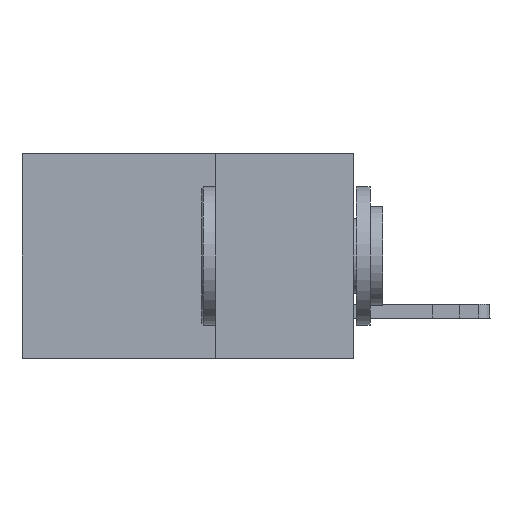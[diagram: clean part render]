
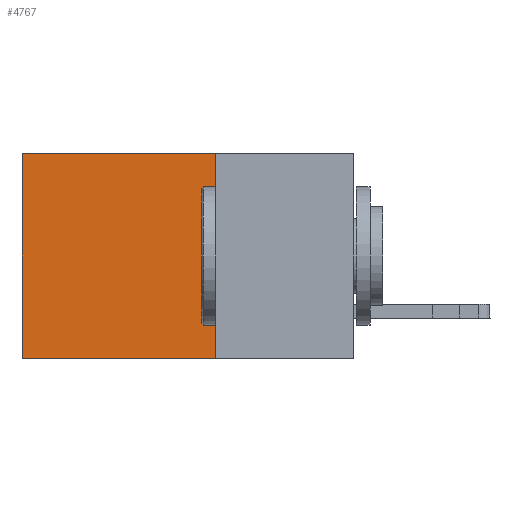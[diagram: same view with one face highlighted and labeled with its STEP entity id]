
A CAD part, left-side view. The second image highlights one B-rep face of the part: STEP entity #4767.
In plain terms, the highlighted planar face has unit normal (-1, 0, 0).
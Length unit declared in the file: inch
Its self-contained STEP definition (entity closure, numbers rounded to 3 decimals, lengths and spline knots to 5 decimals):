
#825 = VERTEX_POINT ( 'NONE', #21535 ) ;
#1037 = DIRECTION ( 'NONE',  ( 1., 0., 0. ) ) ;
#1356 = DIRECTION ( 'NONE',  ( 0., 0., -1. ) ) ;
#3114 = VECTOR ( 'NONE', #20993, 39.37008 ) ;
#3128 = PLANE ( 'NONE',  #12236 ) ;
#3600 = CARTESIAN_POINT ( 'NONE',  ( 0.2875, 0.25, 0. ) ) ;
#4668 = CARTESIAN_POINT ( 'NONE',  ( 0.2875, 0.25, -0.37 ) ) ;
#4767 = ADVANCED_FACE ( 'NONE', ( #8889 ), #3128, .F. ) ;
#4964 = CARTESIAN_POINT ( 'NONE',  ( 0.2875, 0.25, 0. ) ) ;
#5153 = VERTEX_POINT ( 'NONE', #12406 ) ;
#5405 = VERTEX_POINT ( 'NONE', #21095 ) ;
#6827 = VECTOR ( 'NONE', #16389, 39.37008 ) ;
#7416 = VERTEX_POINT ( 'NONE', #22650 ) ;
#8889 = FACE_OUTER_BOUND ( 'NONE', #21487, .T. ) ;
#8951 = EDGE_CURVE ( 'NONE', #5405, #825, #20628, .T. ) ;
#10311 = CARTESIAN_POINT ( 'NONE',  ( 0.2875, 0.25, 0. ) ) ;
#11108 = DIRECTION ( 'NONE',  ( 0., 0., -1. ) ) ;
#12236 = AXIS2_PLACEMENT_3D ( 'NONE', #4964, #1037, #11108 ) ;
#12406 = CARTESIAN_POINT ( 'NONE',  ( 0.2875, 0.6, 0. ) ) ;
#12422 = EDGE_CURVE ( 'NONE', #825, #7416, #25100, .T. ) ;
#12817 = ORIENTED_EDGE ( 'NONE', *, *, #12422, .F. ) ;
#16389 = DIRECTION ( 'NONE',  ( 0., 1., 0. ) ) ;
#17386 = DIRECTION ( 'NONE',  ( 0., 0., -1. ) ) ;
#19432 = CARTESIAN_POINT ( 'NONE',  ( 0.2875, 0.6, 0. ) ) ;
#19577 = VECTOR ( 'NONE', #1356, 39.37008 ) ;
#19586 = ORIENTED_EDGE ( 'NONE', *, *, #22706, .T. ) ;
#20628 = LINE ( 'NONE', #3600, #22531 ) ;
#20993 = DIRECTION ( 'NONE',  ( 0., 1., 0. ) ) ;
#21095 = CARTESIAN_POINT ( 'NONE',  ( 0.2875, 0.25, 0. ) ) ;
#21170 = ORIENTED_EDGE ( 'NONE', *, *, #26031, .T. ) ;
#21487 = EDGE_LOOP ( 'NONE', ( #21170, #12817, #24878, #19586 ) ) ;
#21535 = CARTESIAN_POINT ( 'NONE',  ( 0.2875, 0.25, -0.37 ) ) ;
#22531 = VECTOR ( 'NONE', #17386, 39.37008 ) ;
#22650 = CARTESIAN_POINT ( 'NONE',  ( 0.2875, 0.6, -0.37 ) ) ;
#22706 = EDGE_CURVE ( 'NONE', #5405, #5153, #22882, .T. ) ;
#22882 = LINE ( 'NONE', #10311, #6827 ) ;
#24878 = ORIENTED_EDGE ( 'NONE', *, *, #8951, .F. ) ;
#24939 = LINE ( 'NONE', #19432, #19577 ) ;
#25100 = LINE ( 'NONE', #4668, #3114 ) ;
#26031 = EDGE_CURVE ( 'NONE', #5153, #7416, #24939, .T. ) ;
